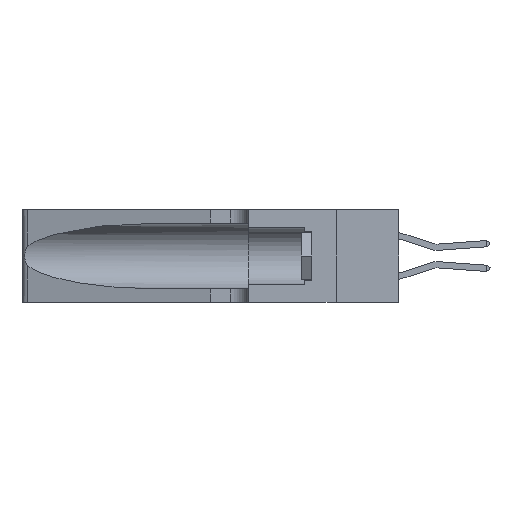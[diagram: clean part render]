
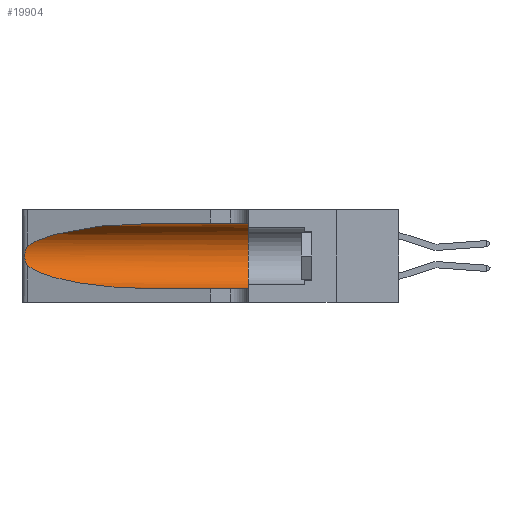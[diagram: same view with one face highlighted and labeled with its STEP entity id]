
A CAD part, left-side view. The second image highlights one B-rep face of the part: STEP entity #19904.
In plain terms, the highlighted cylindrical face has radius 3.308 mm (diameter 6.617 mm), a partial arc.
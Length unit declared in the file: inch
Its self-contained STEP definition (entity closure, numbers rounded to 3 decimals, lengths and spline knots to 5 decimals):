
#150 = CARTESIAN_POINT ( 'NONE',  ( 0.1305, 0.72297, 0.31525 ) ) ;
#623 = EDGE_CURVE ( 'NONE', #17064, #6018, #18968, .T. ) ;
#1251 = CARTESIAN_POINT ( 'NONE',  ( 0.1305, 1.61858, 0.05475 ) ) ;
#1291 = ORIENTED_EDGE ( 'NONE', *, *, #623, .T. ) ;
#1550 = EDGE_CURVE ( 'NONE', #11698, #14145, #19118, .T. ) ;
#1599 = CARTESIAN_POINT ( 'NONE',  ( 0.1305, 0.72297, 0.31525 ) ) ;
#1802 = CARTESIAN_POINT ( 'NONE',  ( 0.25487, 1.22718, 0.14631 ) ) ;
#2489 = ORIENTED_EDGE ( 'NONE', *, *, #18365, .T. ) ;
#3302 = CARTESIAN_POINT ( 'NONE',  ( 0.25487, 1.22718, 0.22369 ) ) ;
#3617 = CARTESIAN_POINT ( 'NONE',  ( 0.25639, 1.23186, 0.15144 ) ) ;
#3795 = CARTESIAN_POINT ( 'NONE',  ( 0.18966, 0.96281, 0.31525 ) ) ;
#5530 = CARTESIAN_POINT ( 'NONE',  ( 0.2373, 1.15595, 0.08982 ) ) ;
#6015 = CARTESIAN_POINT ( 'NONE',  ( 0.25487, 1.22718, 0.22369 ) ) ;
#6018 = VERTEX_POINT ( 'NONE', #14332 ) ;
#6892 = CARTESIAN_POINT ( 'NONE',  ( 0.1305, 1.61858, 0.31525 ) ) ;
#6922 = FACE_OUTER_BOUND ( 'NONE', #19084, .T. ) ;
#8421 = CARTESIAN_POINT ( 'NONE',  ( 0.25487, 1.22718, 0.22369 ) ) ;
#8584 = CARTESIAN_POINT ( 'NONE',  ( 0.26018, 1.23835, 0.19895 ) ) ;
#8704 = CARTESIAN_POINT ( 'NONE',  ( 0.26017, 1.23833, 0.17102 ) ) ;
#8985 = DIRECTION ( 'NONE',  ( 0., -1., 0. ) ) ;
#9005 = EDGE_CURVE ( 'NONE', #14145, #12503, #9681, .T. ) ;
#9566 = CARTESIAN_POINT ( 'NONE',  ( 0.1305, 0.35, 0.185 ) ) ;
#9681 = CIRCLE ( 'NONE', #13054, 0.13025 ) ;
#9752 = CARTESIAN_POINT ( 'NONE',  ( 0.1305, 0.35, 0.05475 ) ) ;
#9802 = ORIENTED_EDGE ( 'NONE', *, *, #1550, .F. ) ;
#10307 = CARTESIAN_POINT ( 'NONE',  ( 0.26075, 1.23896, 0.178 ) ) ;
#10495 = CARTESIAN_POINT ( 'NONE',  ( 0.26075, 1.23896, 0.19203 ) ) ;
#10743 = ORIENTED_EDGE ( 'NONE', *, *, #17634, .T. ) ;
#11698 = VERTEX_POINT ( 'NONE', #150 ) ;
#11755 = DIRECTION ( 'NONE',  ( 0., 0., 1. ) ) ;
#11926 =( BOUNDED_CURVE ( )  B_SPLINE_CURVE ( 3, ( #1599, #3795, #19005, #6015 ),
 .UNSPECIFIED., .F., .F. ) 
 B_SPLINE_CURVE_WITH_KNOTS ( ( 4, 4 ),
 ( 1.5708, 2.84003 ),
 .UNSPECIFIED. ) 
 CURVE ( )  GEOMETRIC_REPRESENTATION_ITEM ( )  RATIONAL_B_SPLINE_CURVE ( ( 1., 0.87, 0.87, 1. ) ) 
 REPRESENTATION_ITEM ( '' )  );
#12175 = CARTESIAN_POINT ( 'NONE',  ( 0.18966, 0.96281, 0.05475 ) ) ;
#12503 = VERTEX_POINT ( 'NONE', #9752 ) ;
#12575 = LINE ( 'NONE', #1251, #23307 ) ;
#13054 = AXIS2_PLACEMENT_3D ( 'NONE', #9566, #24624, #11755 ) ;
#14145 = VERTEX_POINT ( 'NONE', #18444 ) ;
#14332 = CARTESIAN_POINT ( 'NONE',  ( 0.25487, 1.22718, 0.14631 ) ) ;
#15460 = CARTESIAN_POINT ( 'NONE',  ( 0.1305, 1.61858, 0.185 ) ) ;
#16230 = ORIENTED_EDGE ( 'NONE', *, *, #9005, .F. ) ;
#16424 = EDGE_CURVE ( 'NONE', #6018, #18540, #16921, .T. ) ;
#16921 =( BOUNDED_CURVE ( )  B_SPLINE_CURVE ( 3, ( #20727, #5530, #12175, #27147 ),
 .UNSPECIFIED., .F., .F. ) 
 B_SPLINE_CURVE_WITH_KNOTS ( ( 4, 4 ),
 ( 3.44316, 4.71239 ),
 .UNSPECIFIED. ) 
 CURVE ( )  GEOMETRIC_REPRESENTATION_ITEM ( )  RATIONAL_B_SPLINE_CURVE ( ( 1., 0.87, 0.87, 1. ) ) 
 REPRESENTATION_ITEM ( '' )  );
#17064 = VERTEX_POINT ( 'NONE', #3302 ) ;
#17597 = DIRECTION ( 'NONE',  ( 0., 0., -1. ) ) ;
#17634 = EDGE_CURVE ( 'NONE', #18540, #12503, #12575, .T. ) ;
#18365 = EDGE_CURVE ( 'NONE', #11698, #17064, #11926, .T. ) ;
#18444 = CARTESIAN_POINT ( 'NONE',  ( 0.1305, 0.35, 0.31525 ) ) ;
#18455 = VECTOR ( 'NONE', #26141, 39.37008 ) ;
#18540 = VERTEX_POINT ( 'NONE', #19668 ) ;
#18673 = DIRECTION ( 'NONE',  ( 0., -1., 0. ) ) ;
#18968 = B_SPLINE_CURVE_WITH_KNOTS ( 'NONE', 3,
 ( #8421, #27392, #26672, #25707, #26209, #8584, #10495, #10307, #8704, #25640, #25429, #3617, #26189, #1802 ),
 .UNSPECIFIED., .F., .F.,
 ( 4, 2, 2, 2, 2, 2, 4 ),
 ( 0., 0.00027, 0.00053, 0.00107, 0.0016, 0.00187, 0.00214 ),
 .UNSPECIFIED. ) ;
#19005 = CARTESIAN_POINT ( 'NONE',  ( 0.2373, 1.15595, 0.28018 ) ) ;
#19084 = EDGE_LOOP ( 'NONE', ( #2489, #1291, #21016, #10743, #16230, #9802 ) ) ;
#19118 = LINE ( 'NONE', #6892, #18455 ) ;
#19668 = CARTESIAN_POINT ( 'NONE',  ( 0.1305, 0.72297, 0.05475 ) ) ;
#19904 = ADVANCED_FACE ( 'NONE', ( #6922 ), #23507, .F. ) ;
#20554 = AXIS2_PLACEMENT_3D ( 'NONE', #15460, #8985, #17597 ) ;
#20727 = CARTESIAN_POINT ( 'NONE',  ( 0.25487, 1.22718, 0.14631 ) ) ;
#21016 = ORIENTED_EDGE ( 'NONE', *, *, #16424, .T. ) ;
#23307 = VECTOR ( 'NONE', #18673, 39.37008 ) ;
#23507 = CYLINDRICAL_SURFACE ( 'NONE', #20554, 0.13025 ) ;
#24624 = DIRECTION ( 'NONE',  ( 0., 1., 0. ) ) ;
#25429 = CARTESIAN_POINT ( 'NONE',  ( 0.25789, 1.23486, 0.15765 ) ) ;
#25640 = CARTESIAN_POINT ( 'NONE',  ( 0.25856, 1.23593, 0.16098 ) ) ;
#25707 = CARTESIAN_POINT ( 'NONE',  ( 0.25787, 1.23484, 0.2124 ) ) ;
#26141 = DIRECTION ( 'NONE',  ( 0., -1., 0. ) ) ;
#26189 = CARTESIAN_POINT ( 'NONE',  ( 0.25555, 1.22993, 0.14849 ) ) ;
#26209 = CARTESIAN_POINT ( 'NONE',  ( 0.25854, 1.2359, 0.20912 ) ) ;
#26672 = CARTESIAN_POINT ( 'NONE',  ( 0.25639, 1.23184, 0.21858 ) ) ;
#27147 = CARTESIAN_POINT ( 'NONE',  ( 0.1305, 0.72297, 0.05475 ) ) ;
#27392 = CARTESIAN_POINT ( 'NONE',  ( 0.25555, 1.22994, 0.2215 ) ) ;
